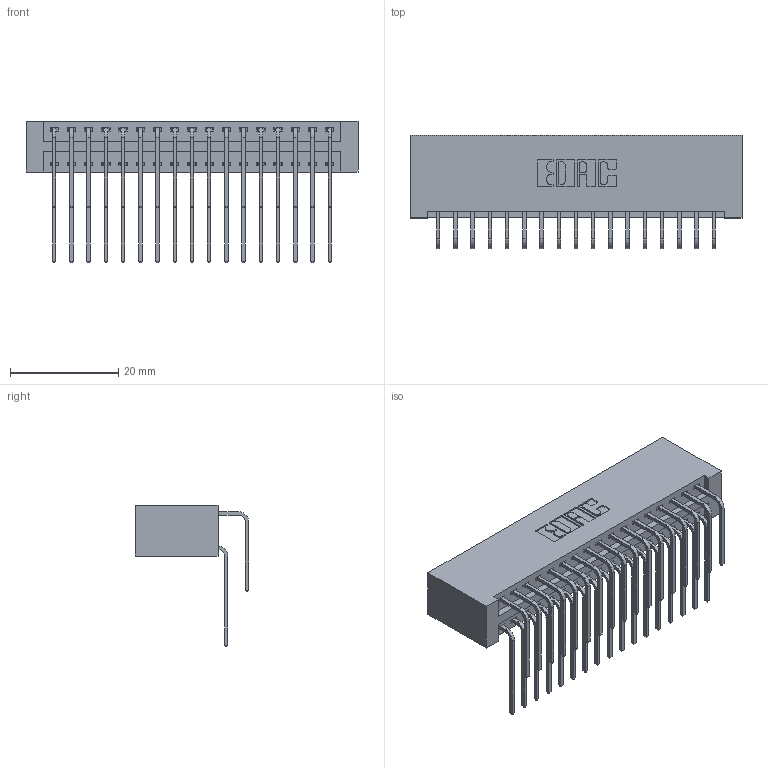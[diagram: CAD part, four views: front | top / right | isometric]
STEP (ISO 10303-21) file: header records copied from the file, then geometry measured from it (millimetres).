
FILE_DESCRIPTION (( 'STEP AP203' ), '1' );
FILE_NAME ('346-034-559-201.STEP', '2022-05-19T20:26:50', ( '' ), ( '' ), 'SwSTEP 2.0', 'SolidWorks 2020', '' );
FILE_SCHEMA (( 'CONFIG_CONTROL_DESIGN' ));
Length unit declared in the file: inch
Products named in the file (4): 346 Part_No Mounting Lugs; 345-292-001_558 559 Tail - 1; 346-034-559-201; 345-292-001_559 Tail - 2
Assembly tree (35 placements, depth 2):
  346-034-559-201
    346 Part_No Mounting Lugs
    345-292-001_558 559 Tail - 1  x17
    345-292-001_559 Tail - 2  x17
Bounding box: 61.21 x 20.89 x 26.16 mm (x, y, z)
Volume: 6544.4 mm3; surface area: 9706.9 mm2
Topology: 35 solids, 35 shells, 1950 faces, 5779 edges, 3806 vertices
Faces by surface type: plane 1330, cylinder 620
Entity records: 15967 total; most frequent: CARTESIAN_POINT 2715, ORIENTED_EDGE 2598, DIRECTION 2411, EDGE_CURVE 1299, LINE 1067, VECTOR 1067, VERTEX_POINT 862, AXIS2_PLACEMENT_3D 672
